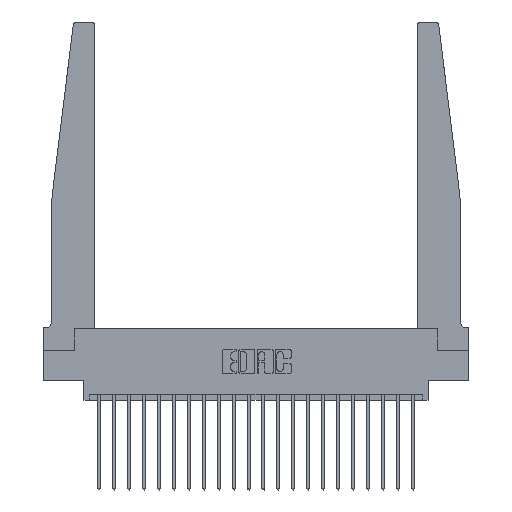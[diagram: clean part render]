
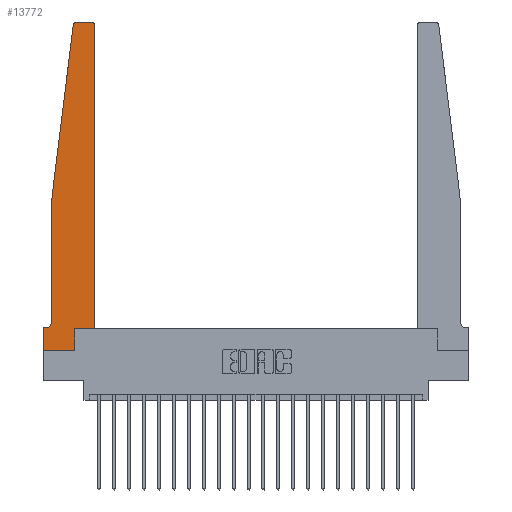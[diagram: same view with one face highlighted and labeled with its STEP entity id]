
A CAD part, top view. The second image highlights one B-rep face of the part: STEP entity #13772.
In plain terms, the highlighted planar face has unit normal (0, 0, 1).
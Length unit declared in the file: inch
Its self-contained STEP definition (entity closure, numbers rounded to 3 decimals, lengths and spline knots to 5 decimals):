
#274 = CARTESIAN_POINT ( 'NONE',  ( 0.24675, 2.72367, 0.37 ) ) ;
#937 = ORIENTED_EDGE ( 'NONE', *, *, #9193, .T. ) ;
#1270 = CARTESIAN_POINT ( 'NONE',  ( 0.27653, 2.75, 0.37 ) ) ;
#1618 = VERTEX_POINT ( 'NONE', #7223 ) ;
#1692 = DIRECTION ( 'NONE',  ( 0., 1., 0. ) ) ;
#2221 = LINE ( 'NONE', #20318, #10741 ) ;
#2259 = LINE ( 'NONE', #14150, #20312 ) ;
#2416 = VERTEX_POINT ( 'NONE', #1270 ) ;
#2482 = CARTESIAN_POINT ( 'NONE',  ( 0.425, 0.18, 0.37 ) ) ;
#2528 = CARTESIAN_POINT ( 'NONE',  ( 0.395, 2.72, 0.37 ) ) ;
#3347 = LINE ( 'NONE', #9897, #20838 ) ;
#3350 = ORIENTED_EDGE ( 'NONE', *, *, #19078, .T. ) ;
#3519 = CARTESIAN_POINT ( 'NONE',  ( 0.2605, 0., 0.37 ) ) ;
#3536 = DIRECTION ( 'NONE',  ( 0., 0., 1. ) ) ;
#3749 = VERTEX_POINT ( 'NONE', #11646 ) ;
#3984 = CARTESIAN_POINT ( 'NONE',  ( 0.065, 1.25, 0.37 ) ) ;
#4019 = DIRECTION ( 'NONE',  ( -1., 0., 0. ) ) ;
#4268 = DIRECTION ( 'NONE',  ( 1., 0., 0. ) ) ;
#4468 = AXIS2_PLACEMENT_3D ( 'NONE', #16383, #6262, #18098 ) ;
#4478 = VECTOR ( 'NONE', #19242, 39.37008 ) ;
#4719 = ORIENTED_EDGE ( 'NONE', *, *, #6275, .T. ) ;
#4774 = DIRECTION ( 'NONE',  ( 0., 0., 1. ) ) ;
#5262 = ORIENTED_EDGE ( 'NONE', *, *, #8060, .T. ) ;
#6056 = ORIENTED_EDGE ( 'NONE', *, *, #9780, .T. ) ;
#6085 = CARTESIAN_POINT ( 'NONE',  ( 0.425, 2.72, 0.37 ) ) ;
#6093 = CARTESIAN_POINT ( 'NONE',  ( 0.395, 2.75, 0.37 ) ) ;
#6154 = DIRECTION ( 'NONE',  ( 0., 1., 0. ) ) ;
#6262 = DIRECTION ( 'NONE',  ( 0., 0., -1. ) ) ;
#6275 = EDGE_CURVE ( 'NONE', #21801, #7679, #3347, .T. ) ;
#6278 = AXIS2_PLACEMENT_3D ( 'NONE', #14900, #4774, #16613 ) ;
#6529 = VECTOR ( 'NONE', #6571, 39.37008 ) ;
#6571 = DIRECTION ( 'NONE',  ( 0., -1., 0. ) ) ;
#6712 = VERTEX_POINT ( 'NONE', #6093 ) ;
#6825 = CARTESIAN_POINT ( 'NONE',  ( 0.425, 0.18, 0.37 ) ) ;
#7223 = CARTESIAN_POINT ( 'NONE',  ( 0., 0.1875, 0.37 ) ) ;
#7639 = DIRECTION ( 'NONE',  ( 1., 0., 0. ) ) ;
#7679 = VERTEX_POINT ( 'NONE', #3519 ) ;
#7710 = VECTOR ( 'NONE', #7639, 39.37008 ) ;
#8060 = EDGE_CURVE ( 'NONE', #9382, #15979, #14368, .T. ) ;
#8986 = LINE ( 'NONE', #3984, #4478 ) ;
#9193 = EDGE_CURVE ( 'NONE', #3749, #9361, #21725, .T. ) ;
#9221 = VERTEX_POINT ( 'NONE', #6085 ) ;
#9226 = ORIENTED_EDGE ( 'NONE', *, *, #20117, .T. ) ;
#9361 = VERTEX_POINT ( 'NONE', #6825 ) ;
#9382 = VERTEX_POINT ( 'NONE', #17025 ) ;
#9395 = ORIENTED_EDGE ( 'NONE', *, *, #21702, .T. ) ;
#9716 = EDGE_LOOP ( 'NONE', ( #6056, #11003, #10306, #9766, #5262, #3350, #9395, #4719, #9226, #937, #12429, #13976 ) ) ;
#9766 = ORIENTED_EDGE ( 'NONE', *, *, #19147, .T. ) ;
#9780 = EDGE_CURVE ( 'NONE', #6712, #2416, #15932, .T. ) ;
#9897 = CARTESIAN_POINT ( 'NONE',  ( 0., 0., 0.37 ) ) ;
#10267 = LINE ( 'NONE', #14285, #18738 ) ;
#10306 = ORIENTED_EDGE ( 'NONE', *, *, #16833, .T. ) ;
#10741 = VECTOR ( 'NONE', #1692, 39.37008 ) ;
#11003 = ORIENTED_EDGE ( 'NONE', *, *, #16626, .T. ) ;
#11025 = LINE ( 'NONE', #13300, #6529 ) ;
#11589 = DIRECTION ( 'NONE',  ( 1., 0., 0. ) ) ;
#11646 = CARTESIAN_POINT ( 'NONE',  ( 0.2605, 0.18, 0.37 ) ) ;
#11649 = CARTESIAN_POINT ( 'NONE',  ( 0.015, 0.1875, 0.37 ) ) ;
#12113 = AXIS2_PLACEMENT_3D ( 'NONE', #2528, #14404, #4268 ) ;
#12288 = VECTOR ( 'NONE', #6154, 39.37008 ) ;
#12429 = ORIENTED_EDGE ( 'NONE', *, *, #20971, .T. ) ;
#12713 = CIRCLE ( 'NONE', #18034, 0.03 ) ;
#13300 = CARTESIAN_POINT ( 'NONE',  ( 0., 0., 0.37 ) ) ;
#13492 = VERTEX_POINT ( 'NONE', #274 ) ;
#13623 = FACE_OUTER_BOUND ( 'NONE', #9716, .T. ) ;
#13675 = CARTESIAN_POINT ( 'NONE',  ( 0.27653, 2.72, 0.37 ) ) ;
#13772 = ADVANCED_FACE ( 'NONE', ( #13623 ), #14827, .T. ) ;
#13976 = ORIENTED_EDGE ( 'NONE', *, *, #17889, .T. ) ;
#14150 = CARTESIAN_POINT ( 'NONE',  ( 0.065, 0.1875, 0.37 ) ) ;
#14285 = CARTESIAN_POINT ( 'NONE',  ( 0.065, 1.25, 0.37 ) ) ;
#14368 = CIRCLE ( 'NONE', #4468, 0.05 ) ;
#14404 = DIRECTION ( 'NONE',  ( 0., 0., 1. ) ) ;
#14827 = PLANE ( 'NONE',  #6278 ) ;
#14900 = CARTESIAN_POINT ( 'NONE',  ( 0., 0.1875, 0.37 ) ) ;
#15378 = DIRECTION ( 'NONE',  ( 1., 0., 0. ) ) ;
#15932 = LINE ( 'NONE', #19460, #19906 ) ;
#15979 = VERTEX_POINT ( 'NONE', #11649 ) ;
#15996 = DIRECTION ( 'NONE',  ( 0., -1., 0. ) ) ;
#16383 = CARTESIAN_POINT ( 'NONE',  ( 0.015, 0.2375, 0.37 ) ) ;
#16613 = DIRECTION ( 'NONE',  ( 1., 0., 0. ) ) ;
#16626 = EDGE_CURVE ( 'NONE', #2416, #13492, #12713, .T. ) ;
#16833 = EDGE_CURVE ( 'NONE', #13492, #19040, #8986, .T. ) ;
#16989 = CARTESIAN_POINT ( 'NONE',  ( 0., 0., 0.37 ) ) ;
#17025 = CARTESIAN_POINT ( 'NONE',  ( 0.065, 0.2375, 0.37 ) ) ;
#17332 = LINE ( 'NONE', #19687, #12288 ) ;
#17889 = EDGE_CURVE ( 'NONE', #9221, #6712, #20326, .T. ) ;
#18034 = AXIS2_PLACEMENT_3D ( 'NONE', #13675, #3536, #15378 ) ;
#18098 = DIRECTION ( 'NONE',  ( -1., 0., 0. ) ) ;
#18738 = VECTOR ( 'NONE', #15996, 39.37008 ) ;
#19040 = VERTEX_POINT ( 'NONE', #19059 ) ;
#19059 = CARTESIAN_POINT ( 'NONE',  ( 0.065, 1.25, 0.37 ) ) ;
#19078 = EDGE_CURVE ( 'NONE', #15979, #1618, #2259, .T. ) ;
#19147 = EDGE_CURVE ( 'NONE', #19040, #9382, #10267, .T. ) ;
#19242 = DIRECTION ( 'NONE',  ( -0.122, -0.992, 0. ) ) ;
#19460 = CARTESIAN_POINT ( 'NONE',  ( 0.25, 2.75, 0.37 ) ) ;
#19687 = CARTESIAN_POINT ( 'NONE',  ( 0.425, 0.18, 0.37 ) ) ;
#19906 = VECTOR ( 'NONE', #21217, 39.37008 ) ;
#20117 = EDGE_CURVE ( 'NONE', #7679, #3749, #2221, .T. ) ;
#20312 = VECTOR ( 'NONE', #4019, 39.37008 ) ;
#20318 = CARTESIAN_POINT ( 'NONE',  ( 0.2605, 0.18, 0.37 ) ) ;
#20326 = CIRCLE ( 'NONE', #12113, 0.03 ) ;
#20838 = VECTOR ( 'NONE', #11589, 39.37008 ) ;
#20971 = EDGE_CURVE ( 'NONE', #9361, #9221, #17332, .T. ) ;
#21217 = DIRECTION ( 'NONE',  ( -1., 0., 0. ) ) ;
#21702 = EDGE_CURVE ( 'NONE', #1618, #21801, #11025, .T. ) ;
#21725 = LINE ( 'NONE', #2482, #7710 ) ;
#21801 = VERTEX_POINT ( 'NONE', #16989 ) ;
